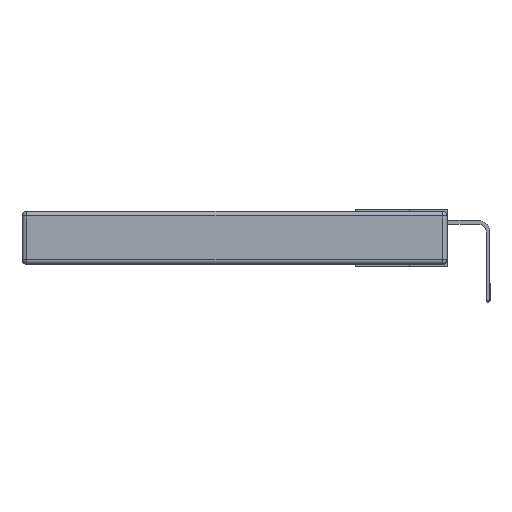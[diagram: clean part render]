
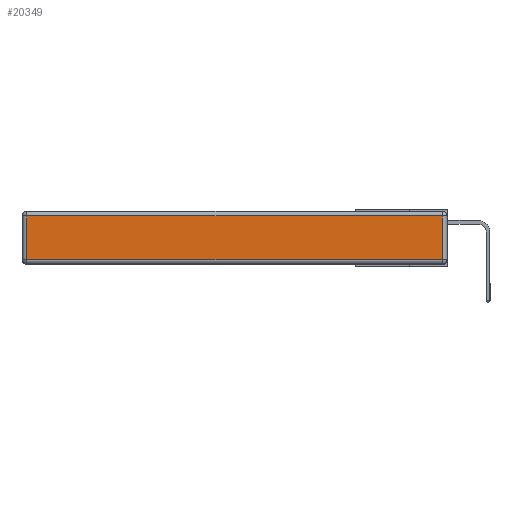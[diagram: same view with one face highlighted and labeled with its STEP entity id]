
A CAD part, left-side view. The second image highlights one B-rep face of the part: STEP entity #20349.
In plain terms, the highlighted planar face has unit normal (-1, 0, 0).
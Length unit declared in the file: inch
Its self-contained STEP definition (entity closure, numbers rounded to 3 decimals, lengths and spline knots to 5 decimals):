
#31 = CARTESIAN_POINT ( 'NONE',  ( 0., 2.75, -0.03 ) ) ;
#163 = CARTESIAN_POINT ( 'NONE',  ( 0., 0., -0.343 ) ) ;
#370 = DIRECTION ( 'NONE',  ( -1., 0., 0. ) ) ;
#592 = VECTOR ( 'NONE', #22253, 39.37008 ) ;
#1262 = VERTEX_POINT ( 'NONE', #9031 ) ;
#3040 = EDGE_LOOP ( 'NONE', ( #20145, #6111, #18703, #13869 ) ) ;
#3424 = CARTESIAN_POINT ( 'NONE',  ( 0., 2.72, -0.03 ) ) ;
#6111 = ORIENTED_EDGE ( 'NONE', *, *, #12100, .T. ) ;
#6535 = CARTESIAN_POINT ( 'NONE',  ( 0., 0.03, -0.313 ) ) ;
#8098 = CARTESIAN_POINT ( 'NONE',  ( 0., 2.72, -0.343 ) ) ;
#9031 = CARTESIAN_POINT ( 'NONE',  ( 0., 0.03, -0.03 ) ) ;
#9111 = EDGE_CURVE ( 'NONE', #22835, #9907, #22796, .T. ) ;
#9385 = DIRECTION ( 'NONE',  ( 0., 0., 1. ) ) ;
#9907 = VERTEX_POINT ( 'NONE', #22711 ) ;
#11181 = VECTOR ( 'NONE', #23913, 39.37008 ) ;
#11217 = CARTESIAN_POINT ( 'NONE',  ( 0., 0.03, -0.343 ) ) ;
#11762 = VECTOR ( 'NONE', #24514, 39.37008 ) ;
#12100 = EDGE_CURVE ( 'NONE', #18896, #1262, #21266, .T. ) ;
#12582 = CARTESIAN_POINT ( 'NONE',  ( 0., 0., -0.313 ) ) ;
#12764 = LINE ( 'NONE', #31, #11762 ) ;
#12824 = FACE_OUTER_BOUND ( 'NONE', #3040, .T. ) ;
#13869 = ORIENTED_EDGE ( 'NONE', *, *, #9111, .T. ) ;
#14579 = EDGE_CURVE ( 'NONE', #9907, #18896, #17044, .T. ) ;
#17044 = LINE ( 'NONE', #12582, #11181 ) ;
#18403 = EDGE_CURVE ( 'NONE', #1262, #22835, #12764, .T. ) ;
#18703 = ORIENTED_EDGE ( 'NONE', *, *, #18403, .T. ) ;
#18896 = VERTEX_POINT ( 'NONE', #6535 ) ;
#20041 = VECTOR ( 'NONE', #23748, 39.37008 ) ;
#20145 = ORIENTED_EDGE ( 'NONE', *, *, #14579, .T. ) ;
#20349 = ADVANCED_FACE ( 'NONE', ( #12824 ), #26793, .T. ) ;
#21266 = LINE ( 'NONE', #11217, #592 ) ;
#22253 = DIRECTION ( 'NONE',  ( 0., 0., 1. ) ) ;
#22711 = CARTESIAN_POINT ( 'NONE',  ( 0., 2.72, -0.313 ) ) ;
#22796 = LINE ( 'NONE', #8098, #20041 ) ;
#22835 = VERTEX_POINT ( 'NONE', #3424 ) ;
#23748 = DIRECTION ( 'NONE',  ( 0., 0., -1. ) ) ;
#23913 = DIRECTION ( 'NONE',  ( 0., -1., 0. ) ) ;
#24489 = AXIS2_PLACEMENT_3D ( 'NONE', #163, #370, #9385 ) ;
#24514 = DIRECTION ( 'NONE',  ( 0., 1., 0. ) ) ;
#26793 = PLANE ( 'NONE',  #24489 ) ;
